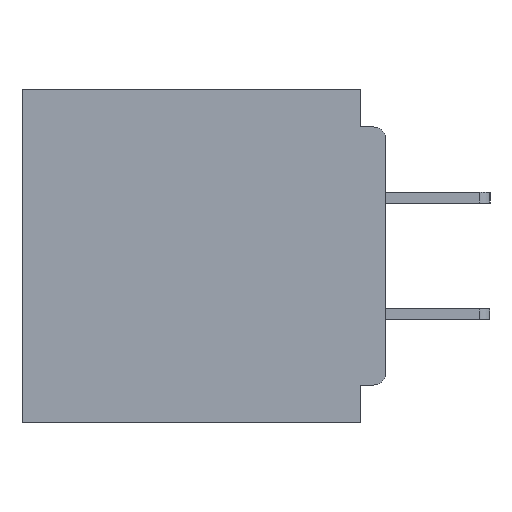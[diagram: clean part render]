
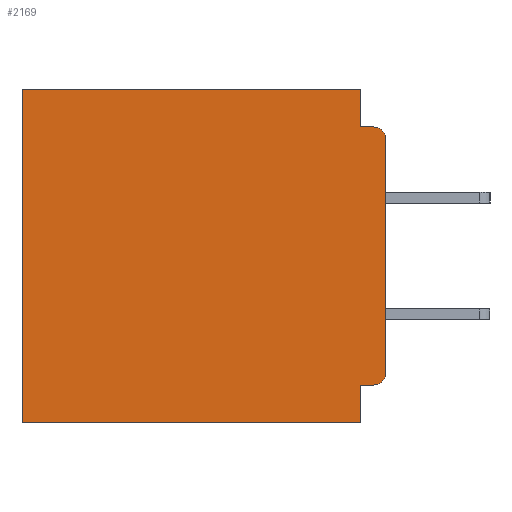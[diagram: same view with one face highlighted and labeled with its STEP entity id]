
A CAD part, left-side view. The second image highlights one B-rep face of the part: STEP entity #2169.
In plain terms, the highlighted planar face has unit normal (-1, 0, 0).
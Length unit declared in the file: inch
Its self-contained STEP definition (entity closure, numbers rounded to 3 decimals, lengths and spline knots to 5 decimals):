
#512 = EDGE_CURVE ( 'NONE', #4522, #40928, #2916, .T. ) ;
#587 = EDGE_LOOP ( 'NONE', ( #14781, #17035, #8673, #20398, #33288, #15379, #44882, #36633, #30507, #12605 ) ) ;
#632 = DIRECTION ( 'NONE',  ( 0., 0., -1. ) ) ;
#1549 = DIRECTION ( 'NONE',  ( 0., 1., 0. ) ) ;
#2169 = ADVANCED_FACE ( 'NONE', ( #44434 ), #7423, .F. ) ;
#2581 = EDGE_CURVE ( 'NONE', #19288, #43535, #39465, .T. ) ;
#2632 = DIRECTION ( 'NONE',  ( 0., 0., -1. ) ) ;
#2916 = LINE ( 'NONE', #17426, #30336 ) ;
#4522 = VERTEX_POINT ( 'NONE', #13900 ) ;
#5626 = AXIS2_PLACEMENT_3D ( 'NONE', #45340, #24025, #2632 ) ;
#5771 = CARTESIAN_POINT ( 'NONE',  ( 0.3, 0.031, 0. ) ) ;
#7399 = EDGE_CURVE ( 'NONE', #32814, #24987, #14961, .T. ) ;
#7423 = PLANE ( 'NONE',  #34825 ) ;
#7857 = CARTESIAN_POINT ( 'NONE',  ( 0.3, 0., -0.34 ) ) ;
#8144 = VERTEX_POINT ( 'NONE', #5771 ) ;
#8673 = ORIENTED_EDGE ( 'NONE', *, *, #26563, .F. ) ;
#10121 = VERTEX_POINT ( 'NONE', #35045 ) ;
#12193 = VECTOR ( 'NONE', #35913, 39.37008 ) ;
#12605 = ORIENTED_EDGE ( 'NONE', *, *, #39373, .T. ) ;
#13900 = CARTESIAN_POINT ( 'NONE',  ( 0.3, 0.437, 0. ) ) ;
#14781 = ORIENTED_EDGE ( 'NONE', *, *, #45597, .F. ) ;
#14961 = LINE ( 'NONE', #30194, #23977 ) ;
#15379 = ORIENTED_EDGE ( 'NONE', *, *, #512, .T. ) ;
#15390 = VECTOR ( 'NONE', #42232, 39.37008 ) ;
#16981 = DIRECTION ( 'NONE',  ( 0., 0., -1. ) ) ;
#17035 = ORIENTED_EDGE ( 'NONE', *, *, #2581, .T. ) ;
#17426 = CARTESIAN_POINT ( 'NONE',  ( 0.3, 0.437, -0.4 ) ) ;
#18147 = EDGE_CURVE ( 'NONE', #24987, #10121, #37445, .T. ) ;
#18473 = VECTOR ( 'NONE', #31196, 39.37008 ) ;
#19288 = VERTEX_POINT ( 'NONE', #45748 ) ;
#20394 = DIRECTION ( 'NONE',  ( 0., 1., 0. ) ) ;
#20398 = ORIENTED_EDGE ( 'NONE', *, *, #20524, .F. ) ;
#20524 = EDGE_CURVE ( 'NONE', #8144, #30401, #34177, .T. ) ;
#20989 = CARTESIAN_POINT ( 'NONE',  ( 0.3, 0.015, -0.355 ) ) ;
#21043 = CARTESIAN_POINT ( 'NONE',  ( 0.3, 0.031, -0.045 ) ) ;
#21670 = LINE ( 'NONE', #39480, #12193 ) ;
#23977 = VECTOR ( 'NONE', #1549, 39.37008 ) ;
#24025 = DIRECTION ( 'NONE',  ( -1., 0., 0. ) ) ;
#24660 = VECTOR ( 'NONE', #31405, 39.37008 ) ;
#24987 = VERTEX_POINT ( 'NONE', #26846 ) ;
#25795 = CARTESIAN_POINT ( 'NONE',  ( 0.3, 0.437, -0.4 ) ) ;
#26286 = DIRECTION ( 'NONE',  ( 0., 0., -1. ) ) ;
#26334 = DIRECTION ( 'NONE',  ( -1., 0., 0. ) ) ;
#26541 = CARTESIAN_POINT ( 'NONE',  ( 0.3, 0.015, -0.06 ) ) ;
#26563 = EDGE_CURVE ( 'NONE', #30401, #43535, #21670, .T. ) ;
#26846 = CARTESIAN_POINT ( 'NONE',  ( 0.3, 0.031, -0.355 ) ) ;
#27611 = CARTESIAN_POINT ( 'NONE',  ( 0.3, 0.031, -0.4 ) ) ;
#27808 = CARTESIAN_POINT ( 'NONE',  ( 0.3, 0.031, 0. ) ) ;
#30194 = CARTESIAN_POINT ( 'NONE',  ( 0.3, 0., -0.355 ) ) ;
#30336 = VECTOR ( 'NONE', #16981, 39.37008 ) ;
#30401 = VERTEX_POINT ( 'NONE', #21043 ) ;
#30507 = ORIENTED_EDGE ( 'NONE', *, *, #7399, .F. ) ;
#31196 = DIRECTION ( 'NONE',  ( 0., 0., -1. ) ) ;
#31405 = DIRECTION ( 'NONE',  ( 0., 0., -1. ) ) ;
#32814 = VERTEX_POINT ( 'NONE', #20989 ) ;
#32932 = CARTESIAN_POINT ( 'NONE',  ( 0.3, 0., -0.4 ) ) ;
#33012 = CIRCLE ( 'NONE', #5626, 0.015 ) ;
#33288 = ORIENTED_EDGE ( 'NONE', *, *, #46019, .T. ) ;
#34177 = LINE ( 'NONE', #27808, #24660 ) ;
#34356 = VECTOR ( 'NONE', #20394, 39.37008 ) ;
#34825 = AXIS2_PLACEMENT_3D ( 'NONE', #32932, #41121, #632 ) ;
#35045 = CARTESIAN_POINT ( 'NONE',  ( 0.3, 0.031, -0.4 ) ) ;
#35504 = LINE ( 'NONE', #38661, #15390 ) ;
#35913 = DIRECTION ( 'NONE',  ( 0., -1., 0. ) ) ;
#36633 = ORIENTED_EDGE ( 'NONE', *, *, #18147, .F. ) ;
#36728 = CARTESIAN_POINT ( 'NONE',  ( 0.3, 0.015, -0.045 ) ) ;
#37445 = LINE ( 'NONE', #27611, #18473 ) ;
#38016 = DIRECTION ( 'NONE',  ( 0., 1., 0. ) ) ;
#38409 = VECTOR ( 'NONE', #38016, 39.37008 ) ;
#38661 = CARTESIAN_POINT ( 'NONE',  ( 0.3, 0., -0.4 ) ) ;
#39031 = VERTEX_POINT ( 'NONE', #7857 ) ;
#39373 = EDGE_CURVE ( 'NONE', #32814, #39031, #33012, .T. ) ;
#39465 = CIRCLE ( 'NONE', #43416, 0.015 ) ;
#39480 = CARTESIAN_POINT ( 'NONE',  ( 0.3, 0., -0.045 ) ) ;
#39519 = LINE ( 'NONE', #44956, #38409 ) ;
#40928 = VERTEX_POINT ( 'NONE', #25795 ) ;
#41121 = DIRECTION ( 'NONE',  ( 1., 0., 0. ) ) ;
#41752 = CARTESIAN_POINT ( 'NONE',  ( 0.3, 0., 0. ) ) ;
#42232 = DIRECTION ( 'NONE',  ( 0., 0., -1. ) ) ;
#43416 = AXIS2_PLACEMENT_3D ( 'NONE', #26541, #26334, #26286 ) ;
#43535 = VERTEX_POINT ( 'NONE', #36728 ) ;
#43755 = LINE ( 'NONE', #41752, #34356 ) ;
#44355 = EDGE_CURVE ( 'NONE', #10121, #40928, #39519, .T. ) ;
#44434 = FACE_OUTER_BOUND ( 'NONE', #587, .T. ) ;
#44882 = ORIENTED_EDGE ( 'NONE', *, *, #44355, .F. ) ;
#44956 = CARTESIAN_POINT ( 'NONE',  ( 0.3, 0., -0.4 ) ) ;
#45340 = CARTESIAN_POINT ( 'NONE',  ( 0.3, 0.015, -0.34 ) ) ;
#45597 = EDGE_CURVE ( 'NONE', #19288, #39031, #35504, .T. ) ;
#45748 = CARTESIAN_POINT ( 'NONE',  ( 0.3, 0., -0.06 ) ) ;
#46019 = EDGE_CURVE ( 'NONE', #8144, #4522, #43755, .T. ) ;
